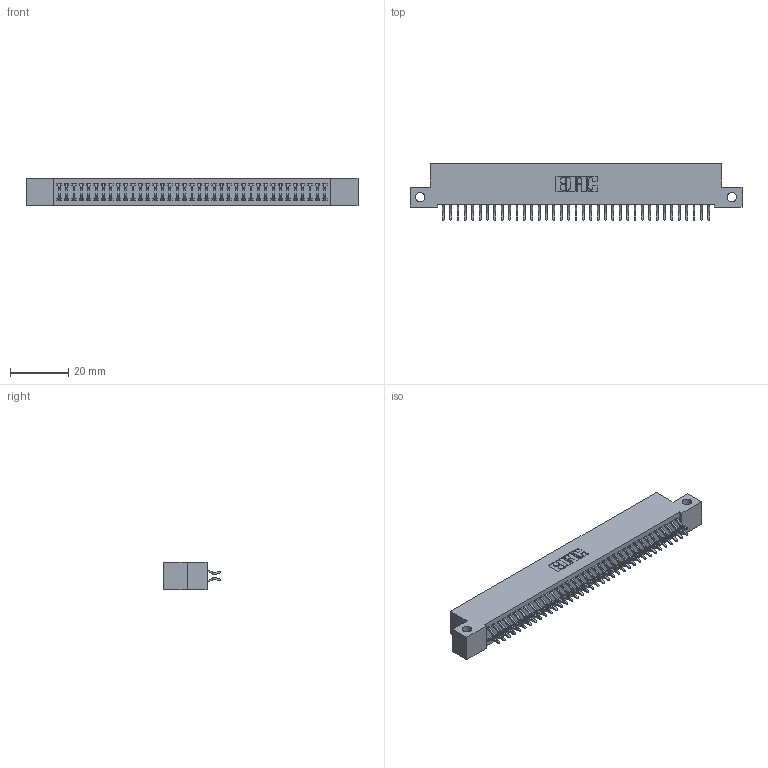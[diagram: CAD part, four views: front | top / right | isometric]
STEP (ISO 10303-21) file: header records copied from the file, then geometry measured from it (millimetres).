
FILE_DESCRIPTION (( 'STEP AP203' ), '1' );
FILE_NAME ('342-074-556-212.STEP', '2019-10-03T17:27:23', ( '' ), ( '' ), 'SwSTEP 2.0', 'SolidWorks 2016', '' );
FILE_SCHEMA (( 'CONFIG_CONTROL_DESIGN' ));
Length unit declared in the file: inch
Products named in the file (3): 342 Part_Side Mount; 345-292-001_556 Tail; 342-074-556-212
Assembly tree (75 placements, depth 2):
  342-074-556-212
    342 Part_Side Mount
    345-292-001_556 Tail  x74
Bounding box: 114.3 x 19.58 x 9.4 mm (x, y, z)
Volume: 10170.4 mm3; surface area: 16200.1 mm2
Topology: 75 solids, 75 shells, 4402 faces, 13101 edges, 8634 vertices
Faces by surface type: plane 3026, cylinder 1376
Entity records: 24541 total; most frequent: CARTESIAN_POINT 4086, ORIENTED_EDGE 4010, DIRECTION 3489, EDGE_CURVE 2005, VECTOR 1869, LINE 1869, VERTEX_POINT 1334, AXIS2_PLACEMENT_3D 810
